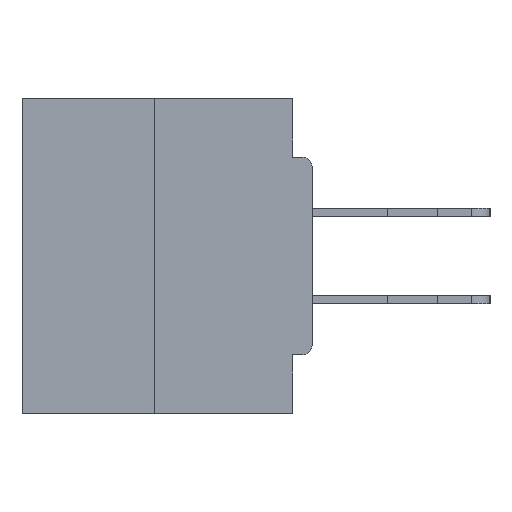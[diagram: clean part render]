
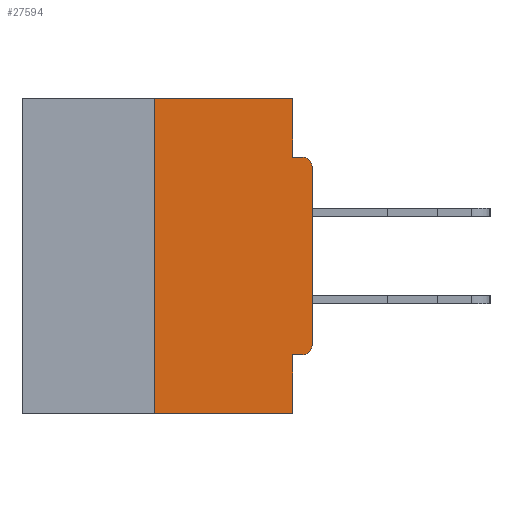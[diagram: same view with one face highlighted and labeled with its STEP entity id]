
A CAD part, left-side view. The second image highlights one B-rep face of the part: STEP entity #27594.
In plain terms, the highlighted planar face has unit normal (-1, 0, 0).
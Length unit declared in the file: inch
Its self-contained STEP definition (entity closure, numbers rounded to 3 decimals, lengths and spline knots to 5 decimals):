
#1 = DIRECTION ( 'NONE',  ( 0., 0., -1. ) ) ;
#443 = DIRECTION ( 'NONE',  ( 0., -1., 0. ) ) ;
#1660 = DIRECTION ( 'NONE',  ( 0., 0., -1. ) ) ;
#1746 = CARTESIAN_POINT ( 'NONE',  ( 0., 0.25, -0.5 ) ) ;
#2827 = CARTESIAN_POINT ( 'NONE',  ( 0., 0.031, -0.5 ) ) ;
#3310 = ORIENTED_EDGE ( 'NONE', *, *, #29715, .F. ) ;
#3544 = ORIENTED_EDGE ( 'NONE', *, *, #4678, .F. ) ;
#3825 = DIRECTION ( 'NONE',  ( 0., 1., 0. ) ) ;
#4495 = CARTESIAN_POINT ( 'NONE',  ( 0., 0.015, -0.0935 ) ) ;
#4555 = ORIENTED_EDGE ( 'NONE', *, *, #22899, .F. ) ;
#4678 = EDGE_CURVE ( 'NONE', #7418, #14457, #5659, .T. ) ;
#5065 = CARTESIAN_POINT ( 'NONE',  ( 0., 0.031, -0.0935 ) ) ;
#5106 = EDGE_LOOP ( 'NONE', ( #23962, #31786, #21967, #3544, #3310, #9927, #28153, #7238, #28097, #4555 ) ) ;
#5211 = VERTEX_POINT ( 'NONE', #4495 ) ;
#5340 = EDGE_CURVE ( 'NONE', #17421, #13960, #14482, .T. ) ;
#5386 = AXIS2_PLACEMENT_3D ( 'NONE', #7320, #18824, #1660 ) ;
#5516 = CARTESIAN_POINT ( 'NONE',  ( 0., 0., 0. ) ) ;
#5659 = LINE ( 'NONE', #2827, #36887 ) ;
#6350 = CARTESIAN_POINT ( 'NONE',  ( 0., 0.25, 0. ) ) ;
#6393 = CARTESIAN_POINT ( 'NONE',  ( 0., 0.25, 0. ) ) ;
#6473 = EDGE_CURVE ( 'NONE', #17623, #5211, #21647, .T. ) ;
#7238 = ORIENTED_EDGE ( 'NONE', *, *, #6473, .T. ) ;
#7302 = VECTOR ( 'NONE', #3825, 39.37008 ) ;
#7320 = CARTESIAN_POINT ( 'NONE',  ( 0., 0.015, -0.1085 ) ) ;
#7418 = VERTEX_POINT ( 'NONE', #24741 ) ;
#7770 = DIRECTION ( 'NONE',  ( 0., -1., 0. ) ) ;
#8100 = CARTESIAN_POINT ( 'NONE',  ( 0., 0.46, 0. ) ) ;
#8196 = CARTESIAN_POINT ( 'NONE',  ( 0., 0.031, -0.5 ) ) ;
#9927 = ORIENTED_EDGE ( 'NONE', *, *, #5340, .T. ) ;
#10508 = CARTESIAN_POINT ( 'NONE',  ( 0., 0.015, -0.3915 ) ) ;
#10732 = DIRECTION ( 'NONE',  ( 0., -1., 0. ) ) ;
#11692 = DIRECTION ( 'NONE',  ( 1., 0., 0. ) ) ;
#12101 = VERTEX_POINT ( 'NONE', #6350 ) ;
#12299 = CARTESIAN_POINT ( 'NONE',  ( 0., 0., -0.4065 ) ) ;
#13960 = VERTEX_POINT ( 'NONE', #18622 ) ;
#14400 = LINE ( 'NONE', #29127, #20828 ) ;
#14457 = VERTEX_POINT ( 'NONE', #8196 ) ;
#14482 = CIRCLE ( 'NONE', #19308, 0.015 ) ;
#14894 = EDGE_CURVE ( 'NONE', #33265, #5211, #33625, .T. ) ;
#16111 = VECTOR ( 'NONE', #7770, 39.37008 ) ;
#17171 = DIRECTION ( 'NONE',  ( 0., 0., -1. ) ) ;
#17421 = VERTEX_POINT ( 'NONE', #33770 ) ;
#17623 = VERTEX_POINT ( 'NONE', #18254 ) ;
#17893 = DIRECTION ( 'NONE',  ( 0., 0., 1. ) ) ;
#18254 = CARTESIAN_POINT ( 'NONE',  ( 0., 0., -0.1085 ) ) ;
#18622 = CARTESIAN_POINT ( 'NONE',  ( 0., 0., -0.3915 ) ) ;
#18824 = DIRECTION ( 'NONE',  ( -1., 0., 0. ) ) ;
#19308 = AXIS2_PLACEMENT_3D ( 'NONE', #10508, #22194, #19371 ) ;
#19371 = DIRECTION ( 'NONE',  ( 0., 0., -1. ) ) ;
#20438 = CARTESIAN_POINT ( 'NONE',  ( 0., 0.031, 0. ) ) ;
#20828 = VECTOR ( 'NONE', #443, 39.37008 ) ;
#21537 = LINE ( 'NONE', #12299, #7302 ) ;
#21647 = CIRCLE ( 'NONE', #5386, 0.015 ) ;
#21967 = ORIENTED_EDGE ( 'NONE', *, *, #22957, .T. ) ;
#22194 = DIRECTION ( 'NONE',  ( -1., 0., 0. ) ) ;
#22425 = EDGE_CURVE ( 'NONE', #12101, #30034, #31674, .T. ) ;
#22899 = EDGE_CURVE ( 'NONE', #30034, #33265, #28757, .T. ) ;
#22957 = EDGE_CURVE ( 'NONE', #23139, #14457, #14400, .T. ) ;
#23139 = VERTEX_POINT ( 'NONE', #1746 ) ;
#23962 = ORIENTED_EDGE ( 'NONE', *, *, #22425, .F. ) ;
#23970 = EDGE_CURVE ( 'NONE', #23139, #12101, #29416, .T. ) ;
#24741 = CARTESIAN_POINT ( 'NONE',  ( 0., 0.031, -0.4065 ) ) ;
#25054 = VECTOR ( 'NONE', #31949, 39.37008 ) ;
#25837 = FACE_OUTER_BOUND ( 'NONE', #5106, .T. ) ;
#26036 = CARTESIAN_POINT ( 'NONE',  ( 0., 0.46, 0. ) ) ;
#26425 = AXIS2_PLACEMENT_3D ( 'NONE', #26036, #11692, #1 ) ;
#27594 = ADVANCED_FACE ( 'NONE', ( #25837 ), #34739, .F. ) ;
#28037 = VECTOR ( 'NONE', #10732, 39.37008 ) ;
#28097 = ORIENTED_EDGE ( 'NONE', *, *, #14894, .F. ) ;
#28153 = ORIENTED_EDGE ( 'NONE', *, *, #33690, .T. ) ;
#28316 = CARTESIAN_POINT ( 'NONE',  ( 0., 0.031, 0. ) ) ;
#28757 = LINE ( 'NONE', #20438, #25054 ) ;
#29127 = CARTESIAN_POINT ( 'NONE',  ( 0., 0.46, -0.5 ) ) ;
#29416 = LINE ( 'NONE', #6393, #31743 ) ;
#29715 = EDGE_CURVE ( 'NONE', #17421, #7418, #21537, .T. ) ;
#30034 = VERTEX_POINT ( 'NONE', #28316 ) ;
#31674 = LINE ( 'NONE', #8100, #28037 ) ;
#31743 = VECTOR ( 'NONE', #17893, 39.37008 ) ;
#31746 = DIRECTION ( 'NONE',  ( 0., 0., 1. ) ) ;
#31786 = ORIENTED_EDGE ( 'NONE', *, *, #23970, .F. ) ;
#31949 = DIRECTION ( 'NONE',  ( 0., 0., -1. ) ) ;
#32543 = VECTOR ( 'NONE', #31746, 39.37008 ) ;
#33255 = CARTESIAN_POINT ( 'NONE',  ( 0., 0., -0.0935 ) ) ;
#33265 = VERTEX_POINT ( 'NONE', #5065 ) ;
#33625 = LINE ( 'NONE', #33255, #16111 ) ;
#33690 = EDGE_CURVE ( 'NONE', #13960, #17623, #37222, .T. ) ;
#33770 = CARTESIAN_POINT ( 'NONE',  ( 0., 0.015, -0.4065 ) ) ;
#34739 = PLANE ( 'NONE',  #26425 ) ;
#36887 = VECTOR ( 'NONE', #17171, 39.37008 ) ;
#37222 = LINE ( 'NONE', #5516, #32543 ) ;
